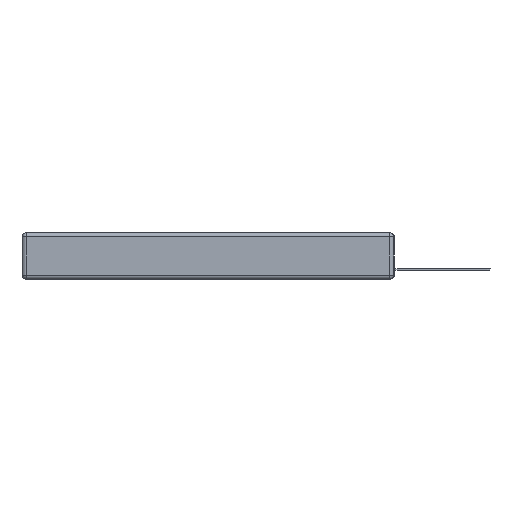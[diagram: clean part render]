
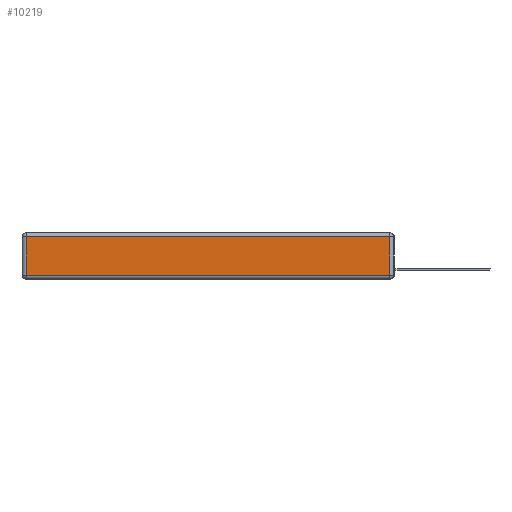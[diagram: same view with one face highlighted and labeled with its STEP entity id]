
A CAD part, left-side view. The second image highlights one B-rep face of the part: STEP entity #10219.
In plain terms, the highlighted planar face has unit normal (-1, 0, 0).
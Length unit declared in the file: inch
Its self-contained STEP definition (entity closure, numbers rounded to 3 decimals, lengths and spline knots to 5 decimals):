
#171 = DIRECTION ( 'NONE',  ( 0., 0., 1. ) ) ;
#888 = ORIENTED_EDGE ( 'NONE', *, *, #16025, .T. ) ;
#1047 = CARTESIAN_POINT ( 'NONE',  ( 0., 2.72, -0.313 ) ) ;
#1079 = VECTOR ( 'NONE', #17511, 39.37008 ) ;
#1133 = VECTOR ( 'NONE', #5438, 39.37008 ) ;
#1322 = CARTESIAN_POINT ( 'NONE',  ( 0., 0.03, -0.313 ) ) ;
#1537 = CARTESIAN_POINT ( 'NONE',  ( 0., 2.72, -0.343 ) ) ;
#2192 = CARTESIAN_POINT ( 'NONE',  ( 0., 0., -0.343 ) ) ;
#2280 = LINE ( 'NONE', #13699, #15134 ) ;
#2810 = VERTEX_POINT ( 'NONE', #1047 ) ;
#5438 = DIRECTION ( 'NONE',  ( 0., -1., 0. ) ) ;
#6948 = VERTEX_POINT ( 'NONE', #8028 ) ;
#7068 = CARTESIAN_POINT ( 'NONE',  ( 0., 0.03, -0.03 ) ) ;
#7590 = EDGE_CURVE ( 'NONE', #6948, #2810, #11290, .T. ) ;
#7747 = LINE ( 'NONE', #14567, #1133 ) ;
#8028 = CARTESIAN_POINT ( 'NONE',  ( 0., 2.72, -0.03 ) ) ;
#8444 = CARTESIAN_POINT ( 'NONE',  ( 0., 2.75, -0.03 ) ) ;
#9219 = EDGE_LOOP ( 'NONE', ( #14345, #17475, #888, #19003 ) ) ;
#10219 = ADVANCED_FACE ( 'NONE', ( #13901 ), #12617, .T. ) ;
#10376 = AXIS2_PLACEMENT_3D ( 'NONE', #2192, #18670, #15875 ) ;
#11290 = LINE ( 'NONE', #1537, #11529 ) ;
#11529 = VECTOR ( 'NONE', #11868, 39.37008 ) ;
#11868 = DIRECTION ( 'NONE',  ( 0., 0., -1. ) ) ;
#12617 = PLANE ( 'NONE',  #10376 ) ;
#13699 = CARTESIAN_POINT ( 'NONE',  ( 0., 0.03, -0.343 ) ) ;
#13806 = VERTEX_POINT ( 'NONE', #7068 ) ;
#13901 = FACE_OUTER_BOUND ( 'NONE', #9219, .T. ) ;
#14345 = ORIENTED_EDGE ( 'NONE', *, *, #14797, .T. ) ;
#14567 = CARTESIAN_POINT ( 'NONE',  ( 0., 0., -0.313 ) ) ;
#14614 = LINE ( 'NONE', #8444, #1079 ) ;
#14797 = EDGE_CURVE ( 'NONE', #2810, #15677, #7747, .T. ) ;
#15093 = EDGE_CURVE ( 'NONE', #15677, #13806, #2280, .T. ) ;
#15134 = VECTOR ( 'NONE', #171, 39.37008 ) ;
#15677 = VERTEX_POINT ( 'NONE', #1322 ) ;
#15875 = DIRECTION ( 'NONE',  ( 0., 0., 1. ) ) ;
#16025 = EDGE_CURVE ( 'NONE', #13806, #6948, #14614, .T. ) ;
#17475 = ORIENTED_EDGE ( 'NONE', *, *, #15093, .T. ) ;
#17511 = DIRECTION ( 'NONE',  ( 0., 1., 0. ) ) ;
#18670 = DIRECTION ( 'NONE',  ( -1., 0., 0. ) ) ;
#19003 = ORIENTED_EDGE ( 'NONE', *, *, #7590, .T. ) ;
